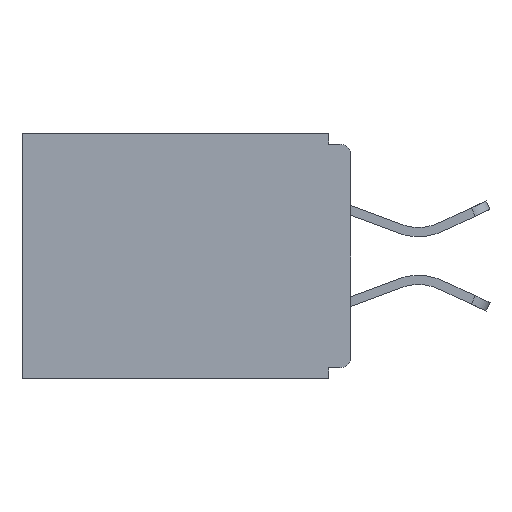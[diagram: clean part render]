
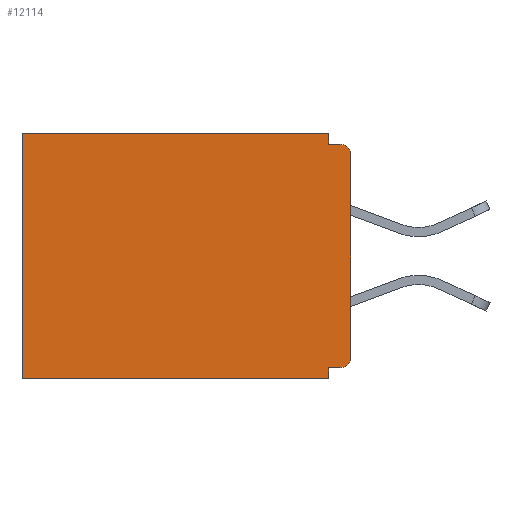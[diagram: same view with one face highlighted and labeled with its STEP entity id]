
A CAD part, left-side view. The second image highlights one B-rep face of the part: STEP entity #12114.
In plain terms, the highlighted planar face has unit normal (-1, 0, 0).
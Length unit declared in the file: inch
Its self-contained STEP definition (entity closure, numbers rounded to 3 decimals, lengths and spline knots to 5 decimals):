
#616 = EDGE_CURVE ( 'NONE', #8940, #15046, #1309, .T. ) ;
#1042 = ORIENTED_EDGE ( 'NONE', *, *, #3506, .T. ) ;
#1103 = DIRECTION ( 'NONE',  ( 0., 0., -1. ) ) ;
#1117 = VECTOR ( 'NONE', #6690, 39.37008 ) ;
#1139 = ORIENTED_EDGE ( 'NONE', *, *, #1231, .F. ) ;
#1231 = EDGE_CURVE ( 'NONE', #9524, #6204, #6291, .T. ) ;
#1296 = CARTESIAN_POINT ( 'NONE',  ( 0.298, 0., -0.328 ) ) ;
#1309 = LINE ( 'NONE', #6235, #9530 ) ;
#1660 = VECTOR ( 'NONE', #8419, 39.37008 ) ;
#2104 = DIRECTION ( 'NONE',  ( -1., 0., 0. ) ) ;
#2246 = ORIENTED_EDGE ( 'NONE', *, *, #12528, .F. ) ;
#2248 = LINE ( 'NONE', #12285, #1660 ) ;
#2310 = EDGE_CURVE ( 'NONE', #8325, #16309, #12286, .T. ) ;
#2346 = VECTOR ( 'NONE', #6114, 39.37008 ) ;
#2388 = DIRECTION ( 'NONE',  ( 1., 0., 0. ) ) ;
#2557 = CIRCLE ( 'NONE', #2645, 0.015 ) ;
#2623 = DIRECTION ( 'NONE',  ( 0., 0., -1. ) ) ;
#2645 = AXIS2_PLACEMENT_3D ( 'NONE', #14858, #2104, #11070 ) ;
#2806 = CARTESIAN_POINT ( 'NONE',  ( 0.298, 0., -0.03 ) ) ;
#2819 = ORIENTED_EDGE ( 'NONE', *, *, #8564, .T. ) ;
#2884 = DIRECTION ( 'NONE',  ( 0., 1., 0. ) ) ;
#3059 = VERTEX_POINT ( 'NONE', #2806 ) ;
#3181 = CARTESIAN_POINT ( 'NONE',  ( 0.298, 0.031, -0.328 ) ) ;
#3243 = CARTESIAN_POINT ( 'NONE',  ( 0.298, 0.015, -0.015 ) ) ;
#3506 = EDGE_CURVE ( 'NONE', #16309, #15046, #15054, .T. ) ;
#3923 = LINE ( 'NONE', #4455, #5538 ) ;
#4015 = VECTOR ( 'NONE', #2623, 39.37008 ) ;
#4328 = CARTESIAN_POINT ( 'NONE',  ( 0.298, 0.015, -0.313 ) ) ;
#4402 = CARTESIAN_POINT ( 'NONE',  ( 0.298, 0.015, -0.328 ) ) ;
#4455 = CARTESIAN_POINT ( 'NONE',  ( 0.298, 0., 0. ) ) ;
#4669 = CARTESIAN_POINT ( 'NONE',  ( 0.298, 0.031, -0.343 ) ) ;
#4757 = CARTESIAN_POINT ( 'NONE',  ( 0.298, 0.031, -0.015 ) ) ;
#4874 = AXIS2_PLACEMENT_3D ( 'NONE', #4328, #11948, #13040 ) ;
#5207 = ORIENTED_EDGE ( 'NONE', *, *, #616, .F. ) ;
#5297 = EDGE_CURVE ( 'NONE', #9911, #9298, #11364, .T. ) ;
#5538 = VECTOR ( 'NONE', #13395, 39.37008 ) ;
#5654 = ORIENTED_EDGE ( 'NONE', *, *, #10802, .F. ) ;
#6083 = AXIS2_PLACEMENT_3D ( 'NONE', #11322, #2388, #1103 ) ;
#6106 = DIRECTION ( 'NONE',  ( 0., 1., 0. ) ) ;
#6114 = DIRECTION ( 'NONE',  ( 0., 0., -1. ) ) ;
#6204 = VERTEX_POINT ( 'NONE', #3181 ) ;
#6235 = CARTESIAN_POINT ( 'NONE',  ( 0.298, 0., -0.343 ) ) ;
#6291 = LINE ( 'NONE', #1296, #13281 ) ;
#6690 = DIRECTION ( 'NONE',  ( 0., -1., 0. ) ) ;
#7397 = CARTESIAN_POINT ( 'NONE',  ( 0.298, 0.46, -0.343 ) ) ;
#8152 = FACE_OUTER_BOUND ( 'NONE', #15385, .T. ) ;
#8325 = VERTEX_POINT ( 'NONE', #10993 ) ;
#8419 = DIRECTION ( 'NONE',  ( 0., 0., -1. ) ) ;
#8564 = EDGE_CURVE ( 'NONE', #9524, #10585, #12608, .T. ) ;
#8651 = CARTESIAN_POINT ( 'NONE',  ( 0.298, 0.46, 0. ) ) ;
#8940 = VERTEX_POINT ( 'NONE', #13760 ) ;
#9207 = CARTESIAN_POINT ( 'NONE',  ( 0.298, 0., 0. ) ) ;
#9298 = VERTEX_POINT ( 'NONE', #3243 ) ;
#9524 = VERTEX_POINT ( 'NONE', #4402 ) ;
#9530 = VECTOR ( 'NONE', #16417, 39.37008 ) ;
#9911 = VERTEX_POINT ( 'NONE', #4757 ) ;
#10345 = ORIENTED_EDGE ( 'NONE', *, *, #2310, .T. ) ;
#10585 = VERTEX_POINT ( 'NONE', #14981 ) ;
#10792 = EDGE_CURVE ( 'NONE', #3059, #9298, #2557, .T. ) ;
#10802 = EDGE_CURVE ( 'NONE', #6204, #8940, #11198, .T. ) ;
#10993 = CARTESIAN_POINT ( 'NONE',  ( 0.298, 0.031, 0. ) ) ;
#11070 = DIRECTION ( 'NONE',  ( 0., 0., -1. ) ) ;
#11198 = LINE ( 'NONE', #4669, #2346 ) ;
#11322 = CARTESIAN_POINT ( 'NONE',  ( 0.298, 0., 0. ) ) ;
#11329 = ORIENTED_EDGE ( 'NONE', *, *, #10792, .T. ) ;
#11364 = LINE ( 'NONE', #13218, #1117 ) ;
#11948 = DIRECTION ( 'NONE',  ( -1., 0., 0. ) ) ;
#12114 = ADVANCED_FACE ( 'NONE', ( #8152 ), #15153, .F. ) ;
#12285 = CARTESIAN_POINT ( 'NONE',  ( 0.298, 0.031, -0.343 ) ) ;
#12286 = LINE ( 'NONE', #9207, #15690 ) ;
#12528 = EDGE_CURVE ( 'NONE', #3059, #10585, #3923, .T. ) ;
#12608 = CIRCLE ( 'NONE', #4874, 0.015 ) ;
#12784 = CARTESIAN_POINT ( 'NONE',  ( 0.298, 0.46, 0. ) ) ;
#13040 = DIRECTION ( 'NONE',  ( 0., 0., -1. ) ) ;
#13108 = ORIENTED_EDGE ( 'NONE', *, *, #14595, .F. ) ;
#13218 = CARTESIAN_POINT ( 'NONE',  ( 0.298, 0., -0.015 ) ) ;
#13281 = VECTOR ( 'NONE', #6106, 39.37008 ) ;
#13357 = ORIENTED_EDGE ( 'NONE', *, *, #5297, .F. ) ;
#13395 = DIRECTION ( 'NONE',  ( 0., 0., -1. ) ) ;
#13760 = CARTESIAN_POINT ( 'NONE',  ( 0.298, 0.031, -0.343 ) ) ;
#14595 = EDGE_CURVE ( 'NONE', #8325, #9911, #2248, .T. ) ;
#14858 = CARTESIAN_POINT ( 'NONE',  ( 0.298, 0.015, -0.03 ) ) ;
#14981 = CARTESIAN_POINT ( 'NONE',  ( 0.298, 0., -0.313 ) ) ;
#15046 = VERTEX_POINT ( 'NONE', #7397 ) ;
#15054 = LINE ( 'NONE', #12784, #4015 ) ;
#15153 = PLANE ( 'NONE',  #6083 ) ;
#15385 = EDGE_LOOP ( 'NONE', ( #11329, #13357, #13108, #10345, #1042, #5207, #5654, #1139, #2819, #2246 ) ) ;
#15690 = VECTOR ( 'NONE', #2884, 39.37008 ) ;
#16309 = VERTEX_POINT ( 'NONE', #8651 ) ;
#16417 = DIRECTION ( 'NONE',  ( 0., 1., 0. ) ) ;
